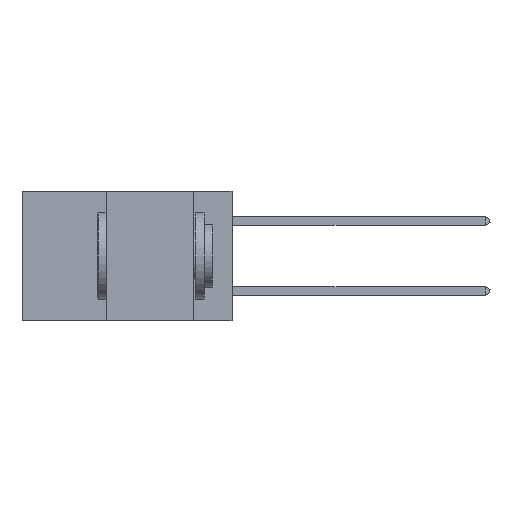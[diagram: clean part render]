
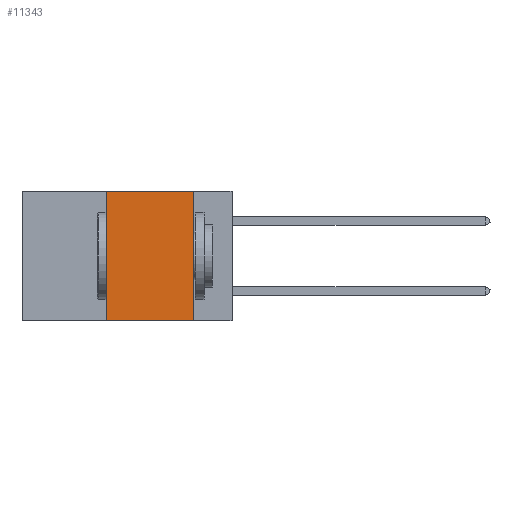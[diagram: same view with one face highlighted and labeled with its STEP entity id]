
A CAD part, left-side view. The second image highlights one B-rep face of the part: STEP entity #11343.
In plain terms, the highlighted planar face has unit normal (-1, 0, 0).
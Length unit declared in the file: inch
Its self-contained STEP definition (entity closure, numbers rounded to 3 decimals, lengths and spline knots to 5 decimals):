
#190 = EDGE_CURVE ( 'NONE', #3747, #12370, #6870, .T. ) ;
#665 = DIRECTION ( 'NONE',  ( 0., -1., 0. ) ) ;
#800 = ORIENTED_EDGE ( 'NONE', *, *, #5459, .F. ) ;
#1065 = DIRECTION ( 'NONE',  ( 0., 0., -1. ) ) ;
#1127 = CARTESIAN_POINT ( 'NONE',  ( 0., 0.6, -0.37 ) ) ;
#1146 = ORIENTED_EDGE ( 'NONE', *, *, #13324, .F. ) ;
#1166 = ORIENTED_EDGE ( 'NONE', *, *, #190, .T. ) ;
#1276 = ORIENTED_EDGE ( 'NONE', *, *, #7991, .F. ) ;
#1566 = LINE ( 'NONE', #8314, #8696 ) ;
#1696 = CARTESIAN_POINT ( 'NONE',  ( 0., 0.36, -0.37 ) ) ;
#2146 = CARTESIAN_POINT ( 'NONE',  ( 0., 0.36, 0. ) ) ;
#2288 = VECTOR ( 'NONE', #10126, 39.37008 ) ;
#2519 = AXIS2_PLACEMENT_3D ( 'NONE', #7477, #8698, #1065 ) ;
#3268 = VERTEX_POINT ( 'NONE', #8630 ) ;
#3442 = VECTOR ( 'NONE', #665, 39.37008 ) ;
#3747 = VERTEX_POINT ( 'NONE', #1696 ) ;
#4265 = LINE ( 'NONE', #12592, #10465 ) ;
#5459 = EDGE_CURVE ( 'NONE', #3747, #11227, #1566, .T. ) ;
#6080 = LINE ( 'NONE', #8929, #2288 ) ;
#6210 = PLANE ( 'NONE',  #2519 ) ;
#6870 = LINE ( 'NONE', #1127, #3442 ) ;
#7477 = CARTESIAN_POINT ( 'NONE',  ( 0., 0.6, 0. ) ) ;
#7991 = EDGE_CURVE ( 'NONE', #3268, #12370, #4265, .T. ) ;
#8257 = EDGE_LOOP ( 'NONE', ( #1276, #1146, #800, #1166 ) ) ;
#8286 = DIRECTION ( 'NONE',  ( 0., 0., 1. ) ) ;
#8314 = CARTESIAN_POINT ( 'NONE',  ( 0., 0.36, 0. ) ) ;
#8630 = CARTESIAN_POINT ( 'NONE',  ( 0., 0.11, 0. ) ) ;
#8696 = VECTOR ( 'NONE', #8286, 39.37008 ) ;
#8698 = DIRECTION ( 'NONE',  ( 1., 0., 0. ) ) ;
#8929 = CARTESIAN_POINT ( 'NONE',  ( 0., 0.6, 0. ) ) ;
#10126 = DIRECTION ( 'NONE',  ( 0., -1., 0. ) ) ;
#10135 = FACE_OUTER_BOUND ( 'NONE', #8257, .T. ) ;
#10465 = VECTOR ( 'NONE', #13792, 39.37008 ) ;
#11227 = VERTEX_POINT ( 'NONE', #2146 ) ;
#11343 = ADVANCED_FACE ( 'NONE', ( #10135 ), #6210, .F. ) ;
#12370 = VERTEX_POINT ( 'NONE', #15465 ) ;
#12592 = CARTESIAN_POINT ( 'NONE',  ( 0., 0.11, 0. ) ) ;
#13324 = EDGE_CURVE ( 'NONE', #11227, #3268, #6080, .T. ) ;
#13792 = DIRECTION ( 'NONE',  ( 0., 0., -1. ) ) ;
#15465 = CARTESIAN_POINT ( 'NONE',  ( 0., 0.11, -0.37 ) ) ;
